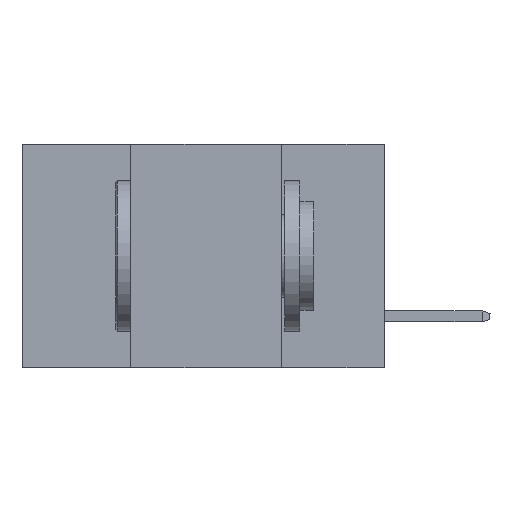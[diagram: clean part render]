
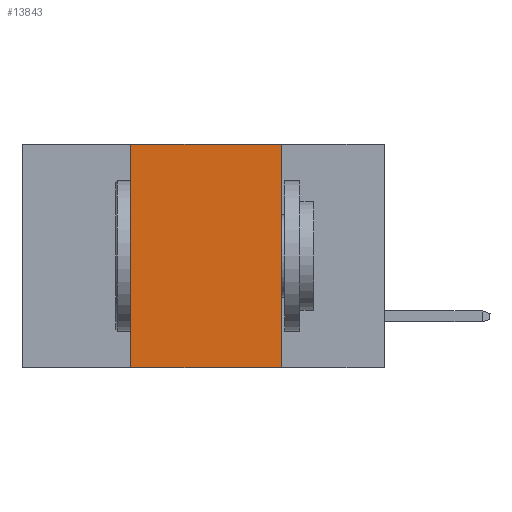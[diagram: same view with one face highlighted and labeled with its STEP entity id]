
A CAD part, left-side view. The second image highlights one B-rep face of the part: STEP entity #13843.
In plain terms, the highlighted planar face has unit normal (-1, 0, 0).
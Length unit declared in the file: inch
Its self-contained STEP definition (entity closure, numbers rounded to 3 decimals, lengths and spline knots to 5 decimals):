
#218 = VERTEX_POINT ( 'NONE', #18339 ) ;
#392 = CARTESIAN_POINT ( 'NONE',  ( 0., 0.17, -0.37 ) ) ;
#2654 = PLANE ( 'NONE',  #20663 ) ;
#4531 = ORIENTED_EDGE ( 'NONE', *, *, #15236, .F. ) ;
#4660 = DIRECTION ( 'NONE',  ( 0., 0., -1. ) ) ;
#4976 = CARTESIAN_POINT ( 'NONE',  ( 0., 0.17, 0. ) ) ;
#5164 = FACE_OUTER_BOUND ( 'NONE', #10422, .T. ) ;
#5809 = LINE ( 'NONE', #9235, #24122 ) ;
#5961 = ORIENTED_EDGE ( 'NONE', *, *, #13995, .F. ) ;
#7018 = ORIENTED_EDGE ( 'NONE', *, *, #12786, .T. ) ;
#7191 = VERTEX_POINT ( 'NONE', #22343 ) ;
#7843 = VECTOR ( 'NONE', #8779, 39.37008 ) ;
#8529 = CARTESIAN_POINT ( 'NONE',  ( 0., 0.6, 0. ) ) ;
#8779 = DIRECTION ( 'NONE',  ( 0., -1., 0. ) ) ;
#9235 = CARTESIAN_POINT ( 'NONE',  ( 0., 0.6, -0.37 ) ) ;
#10422 = EDGE_LOOP ( 'NONE', ( #10737, #4531, #5961, #7018 ) ) ;
#10737 = ORIENTED_EDGE ( 'NONE', *, *, #16407, .F. ) ;
#10939 = CARTESIAN_POINT ( 'NONE',  ( 0., 0.42, -0.37 ) ) ;
#11138 = DIRECTION ( 'NONE',  ( 0., -1., 0. ) ) ;
#11196 = VECTOR ( 'NONE', #21850, 39.37008 ) ;
#11245 = VERTEX_POINT ( 'NONE', #17243 ) ;
#12786 = EDGE_CURVE ( 'NONE', #218, #11245, #5809, .T. ) ;
#12866 = LINE ( 'NONE', #17895, #7843 ) ;
#13843 = ADVANCED_FACE ( 'NONE', ( #5164 ), #2654, .F. ) ;
#13995 = EDGE_CURVE ( 'NONE', #218, #7191, #17712, .T. ) ;
#15236 = EDGE_CURVE ( 'NONE', #7191, #21072, #12866, .T. ) ;
#15966 = DIRECTION ( 'NONE',  ( 1., 0., 0. ) ) ;
#16407 = EDGE_CURVE ( 'NONE', #21072, #11245, #18988, .T. ) ;
#17243 = CARTESIAN_POINT ( 'NONE',  ( 0., 0.17, -0.37 ) ) ;
#17712 = LINE ( 'NONE', #10939, #11196 ) ;
#17895 = CARTESIAN_POINT ( 'NONE',  ( 0., 0.6, 0. ) ) ;
#18339 = CARTESIAN_POINT ( 'NONE',  ( 0., 0.42, -0.37 ) ) ;
#18432 = VECTOR ( 'NONE', #19241, 39.37008 ) ;
#18988 = LINE ( 'NONE', #392, #18432 ) ;
#19241 = DIRECTION ( 'NONE',  ( 0., 0., -1. ) ) ;
#20663 = AXIS2_PLACEMENT_3D ( 'NONE', #8529, #15966, #4660 ) ;
#21072 = VERTEX_POINT ( 'NONE', #4976 ) ;
#21850 = DIRECTION ( 'NONE',  ( 0., 0., 1. ) ) ;
#22343 = CARTESIAN_POINT ( 'NONE',  ( 0., 0.42, 0. ) ) ;
#24122 = VECTOR ( 'NONE', #11138, 39.37008 ) ;
